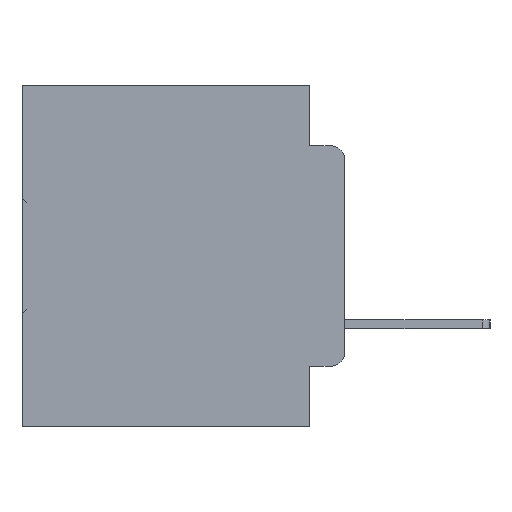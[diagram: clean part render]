
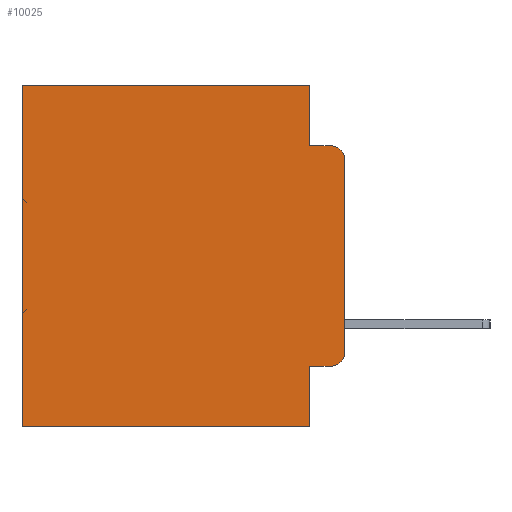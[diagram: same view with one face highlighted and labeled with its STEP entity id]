
A CAD part, left-side view. The second image highlights one B-rep face of the part: STEP entity #10025.
In plain terms, the highlighted planar face has unit normal (-1, 0, 0).
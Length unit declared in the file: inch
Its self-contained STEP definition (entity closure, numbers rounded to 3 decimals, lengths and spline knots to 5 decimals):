
#119 = VECTOR ( 'NONE', #16076, 39.37008 ) ;
#1367 = LINE ( 'NONE', #22593, #15097 ) ;
#1683 = ORIENTED_EDGE ( 'NONE', *, *, #33321, .T. ) ;
#1753 = VECTOR ( 'NONE', #33908, 39.37008 ) ;
#2050 = LINE ( 'NONE', #14993, #29212 ) ;
#2136 = VERTEX_POINT ( 'NONE', #31938 ) ;
#2396 = CARTESIAN_POINT ( 'NONE',  ( 0.298, 0.051, 0. ) ) ;
#2430 = CARTESIAN_POINT ( 'NONE',  ( 0.298, 0., -0.3915 ) ) ;
#2650 = EDGE_CURVE ( 'NONE', #21368, #23569, #29862, .T. ) ;
#2667 = CARTESIAN_POINT ( 'NONE',  ( 0.298, 0.02, -0.3915 ) ) ;
#2844 = CARTESIAN_POINT ( 'NONE',  ( 0.298, 0.02, -0.0885 ) ) ;
#3699 = VERTEX_POINT ( 'NONE', #34596 ) ;
#3704 = ORIENTED_EDGE ( 'NONE', *, *, #12350, .F. ) ;
#4290 = ORIENTED_EDGE ( 'NONE', *, *, #12872, .T. ) ;
#4391 = AXIS2_PLACEMENT_3D ( 'NONE', #24407, #22494, #22463 ) ;
#4908 = CARTESIAN_POINT ( 'NONE',  ( 0.298, 0., 0. ) ) ;
#5102 = LINE ( 'NONE', #25321, #33044 ) ;
#5149 = ORIENTED_EDGE ( 'NONE', *, *, #21770, .T. ) ;
#5300 = CIRCLE ( 'NONE', #31351, 0.02 ) ;
#5384 = DIRECTION ( 'NONE',  ( 0., 0., -1. ) ) ;
#5696 = LINE ( 'NONE', #26697, #12202 ) ;
#6857 = VERTEX_POINT ( 'NONE', #11412 ) ;
#7669 = DIRECTION ( 'NONE',  ( 0., 0., -1. ) ) ;
#7885 = EDGE_CURVE ( 'NONE', #3699, #2136, #5696, .T. ) ;
#9813 = DIRECTION ( 'NONE',  ( 0., 0., -1. ) ) ;
#10025 = ADVANCED_FACE ( 'NONE', ( #14747 ), #21260, .F. ) ;
#10237 = VERTEX_POINT ( 'NONE', #11309 ) ;
#10337 = ORIENTED_EDGE ( 'NONE', *, *, #2650, .T. ) ;
#11114 = LINE ( 'NONE', #20669, #31750 ) ;
#11309 = CARTESIAN_POINT ( 'NONE',  ( 0.298, 0.051, -0.0885 ) ) ;
#11412 = CARTESIAN_POINT ( 'NONE',  ( 0.298, 0.051, -0.4115 ) ) ;
#11608 = EDGE_CURVE ( 'NONE', #10237, #23569, #5102, .T. ) ;
#12202 = VECTOR ( 'NONE', #29378, 39.37008 ) ;
#12350 = EDGE_CURVE ( 'NONE', #21368, #29728, #11114, .T. ) ;
#12792 = VECTOR ( 'NONE', #27076, 39.37008 ) ;
#12872 = EDGE_CURVE ( 'NONE', #24555, #30789, #2050, .T. ) ;
#12930 = ORIENTED_EDGE ( 'NONE', *, *, #31187, .T. ) ;
#14599 = DIRECTION ( 'NONE',  ( 0., -1., 0. ) ) ;
#14747 = FACE_OUTER_BOUND ( 'NONE', #20400, .T. ) ;
#14993 = CARTESIAN_POINT ( 'NONE',  ( 0.298, 0., 0. ) ) ;
#15097 = VECTOR ( 'NONE', #19902, 39.37008 ) ;
#15503 = LINE ( 'NONE', #2396, #119 ) ;
#15614 = AXIS2_PLACEMENT_3D ( 'NONE', #4908, #23988, #7669 ) ;
#16076 = DIRECTION ( 'NONE',  ( 0., 0., -1. ) ) ;
#18052 = CARTESIAN_POINT ( 'NONE',  ( 0.298, 0.473, 0. ) ) ;
#19323 = EDGE_CURVE ( 'NONE', #6857, #3699, #30596, .T. ) ;
#19902 = DIRECTION ( 'NONE',  ( 0., 0., -1. ) ) ;
#20012 = LINE ( 'NONE', #34820, #12792 ) ;
#20400 = EDGE_LOOP ( 'NONE', ( #3704, #10337, #24760, #30603, #4290, #12930, #22666, #31430, #5149, #1683 ) ) ;
#20669 = CARTESIAN_POINT ( 'NONE',  ( 0.298, 0., 0. ) ) ;
#20963 = CARTESIAN_POINT ( 'NONE',  ( 0.298, 0.02, -0.4115 ) ) ;
#21260 = PLANE ( 'NONE',  #15614 ) ;
#21368 = VERTEX_POINT ( 'NONE', #28035 ) ;
#21633 = VERTEX_POINT ( 'NONE', #20963 ) ;
#21754 = DIRECTION ( 'NONE',  ( -1., 0., 0. ) ) ;
#21770 = EDGE_CURVE ( 'NONE', #6857, #21633, #20012, .T. ) ;
#22463 = DIRECTION ( 'NONE',  ( 0., 0., -1. ) ) ;
#22494 = DIRECTION ( 'NONE',  ( -1., 0., 0. ) ) ;
#22593 = CARTESIAN_POINT ( 'NONE',  ( 0.298, 0.473, 0. ) ) ;
#22666 = ORIENTED_EDGE ( 'NONE', *, *, #7885, .F. ) ;
#23101 = CARTESIAN_POINT ( 'NONE',  ( 0.298, 0.051, 0. ) ) ;
#23569 = VERTEX_POINT ( 'NONE', #2844 ) ;
#23988 = DIRECTION ( 'NONE',  ( 1., 0., 0. ) ) ;
#24407 = CARTESIAN_POINT ( 'NONE',  ( 0.298, 0.02, -0.1085 ) ) ;
#24555 = VERTEX_POINT ( 'NONE', #32033 ) ;
#24760 = ORIENTED_EDGE ( 'NONE', *, *, #11608, .F. ) ;
#25321 = CARTESIAN_POINT ( 'NONE',  ( 0.298, 0.051, -0.0885 ) ) ;
#26697 = CARTESIAN_POINT ( 'NONE',  ( 0.298, 0., -0.5 ) ) ;
#27076 = DIRECTION ( 'NONE',  ( 0., -1., 0. ) ) ;
#28035 = CARTESIAN_POINT ( 'NONE',  ( 0.298, 0., -0.1085 ) ) ;
#28374 = DIRECTION ( 'NONE',  ( 0., 1., 0. ) ) ;
#29212 = VECTOR ( 'NONE', #28374, 39.37008 ) ;
#29378 = DIRECTION ( 'NONE',  ( 0., 1., 0. ) ) ;
#29728 = VERTEX_POINT ( 'NONE', #2430 ) ;
#29862 = CIRCLE ( 'NONE', #4391, 0.02 ) ;
#30596 = LINE ( 'NONE', #23101, #1753 ) ;
#30603 = ORIENTED_EDGE ( 'NONE', *, *, #32108, .F. ) ;
#30789 = VERTEX_POINT ( 'NONE', #18052 ) ;
#31187 = EDGE_CURVE ( 'NONE', #30789, #2136, #1367, .T. ) ;
#31351 = AXIS2_PLACEMENT_3D ( 'NONE', #2667, #21754, #5384 ) ;
#31430 = ORIENTED_EDGE ( 'NONE', *, *, #19323, .F. ) ;
#31750 = VECTOR ( 'NONE', #9813, 39.37008 ) ;
#31938 = CARTESIAN_POINT ( 'NONE',  ( 0.298, 0.473, -0.5 ) ) ;
#32033 = CARTESIAN_POINT ( 'NONE',  ( 0.298, 0.051, 0. ) ) ;
#32108 = EDGE_CURVE ( 'NONE', #24555, #10237, #15503, .T. ) ;
#33044 = VECTOR ( 'NONE', #14599, 39.37008 ) ;
#33321 = EDGE_CURVE ( 'NONE', #21633, #29728, #5300, .T. ) ;
#33908 = DIRECTION ( 'NONE',  ( 0., 0., -1. ) ) ;
#34596 = CARTESIAN_POINT ( 'NONE',  ( 0.298, 0.051, -0.5 ) ) ;
#34820 = CARTESIAN_POINT ( 'NONE',  ( 0.298, 0.051, -0.4115 ) ) ;
